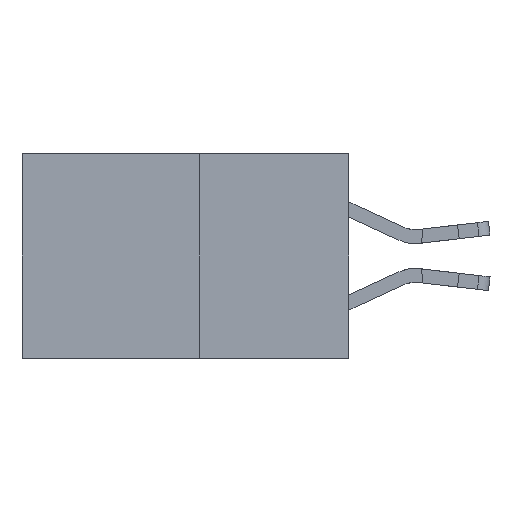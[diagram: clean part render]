
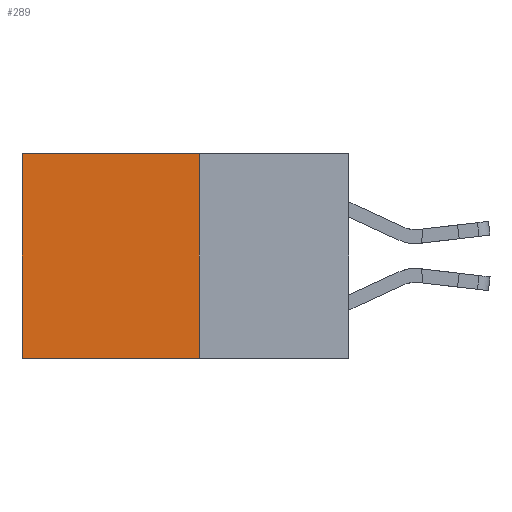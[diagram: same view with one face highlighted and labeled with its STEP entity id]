
A CAD part, left-side view. The second image highlights one B-rep face of the part: STEP entity #289.
In plain terms, the highlighted planar face has unit normal (-1, 0, 0).
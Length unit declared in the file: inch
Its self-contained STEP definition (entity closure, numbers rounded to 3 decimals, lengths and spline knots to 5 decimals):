
#208 = VERTEX_POINT ( 'NONE', #8466 ) ;
#289 = ADVANCED_FACE ( 'NONE', ( #10159 ), #5454, .F. ) ;
#962 = LINE ( 'NONE', #17022, #8165 ) ;
#1034 = VERTEX_POINT ( 'NONE', #6881 ) ;
#1753 = CARTESIAN_POINT ( 'NONE',  ( 0.277, 0.27, 0. ) ) ;
#1842 = EDGE_LOOP ( 'NONE', ( #16858, #6797, #13989, #3428 ) ) ;
#2548 = VECTOR ( 'NONE', #4293, 39.37008 ) ;
#2862 = LINE ( 'NONE', #15820, #6244 ) ;
#3428 = ORIENTED_EDGE ( 'NONE', *, *, #17154, .T. ) ;
#4293 = DIRECTION ( 'NONE',  ( 0., 1., 0. ) ) ;
#4655 = CARTESIAN_POINT ( 'NONE',  ( 0.277, 0.27, -0.37 ) ) ;
#4823 = EDGE_CURVE ( 'NONE', #12731, #208, #9321, .T. ) ;
#5266 = EDGE_CURVE ( 'NONE', #208, #9708, #9752, .T. ) ;
#5454 = PLANE ( 'NONE',  #17862 ) ;
#5995 = CARTESIAN_POINT ( 'NONE',  ( 0.277, 0.59, -0.37 ) ) ;
#6244 = VECTOR ( 'NONE', #11578, 39.37008 ) ;
#6797 = ORIENTED_EDGE ( 'NONE', *, *, #5266, .F. ) ;
#6881 = CARTESIAN_POINT ( 'NONE',  ( 0.277, 0.59, 0. ) ) ;
#7010 = DIRECTION ( 'NONE',  ( 0., 1., 0. ) ) ;
#7699 = DIRECTION ( 'NONE',  ( 1., 0., 0. ) ) ;
#8165 = VECTOR ( 'NONE', #7010, 39.37008 ) ;
#8466 = CARTESIAN_POINT ( 'NONE',  ( 0.277, 0.27, -0.37 ) ) ;
#9321 = LINE ( 'NONE', #14714, #16914 ) ;
#9708 = VERTEX_POINT ( 'NONE', #5995 ) ;
#9752 = LINE ( 'NONE', #4655, #2548 ) ;
#10159 = FACE_OUTER_BOUND ( 'NONE', #1842, .T. ) ;
#11578 = DIRECTION ( 'NONE',  ( 0., 0., -1. ) ) ;
#12731 = VERTEX_POINT ( 'NONE', #1753 ) ;
#13989 = ORIENTED_EDGE ( 'NONE', *, *, #4823, .F. ) ;
#14138 = EDGE_CURVE ( 'NONE', #1034, #9708, #2862, .T. ) ;
#14690 = DIRECTION ( 'NONE',  ( 0., 0., -1. ) ) ;
#14714 = CARTESIAN_POINT ( 'NONE',  ( 0.277, 0.27, -0.37 ) ) ;
#14724 = DIRECTION ( 'NONE',  ( 0., 0., -1. ) ) ;
#15733 = CARTESIAN_POINT ( 'NONE',  ( 0.277, 0.27, -0.37 ) ) ;
#15820 = CARTESIAN_POINT ( 'NONE',  ( 0.277, 0.59, -0.37 ) ) ;
#16858 = ORIENTED_EDGE ( 'NONE', *, *, #14138, .T. ) ;
#16914 = VECTOR ( 'NONE', #14690, 39.37008 ) ;
#17022 = CARTESIAN_POINT ( 'NONE',  ( 0.277, 0.27, 0. ) ) ;
#17154 = EDGE_CURVE ( 'NONE', #12731, #1034, #962, .T. ) ;
#17862 = AXIS2_PLACEMENT_3D ( 'NONE', #15733, #7699, #14724 ) ;
